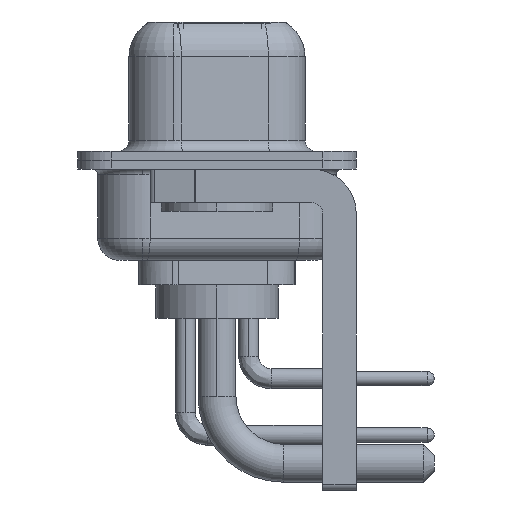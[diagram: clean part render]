
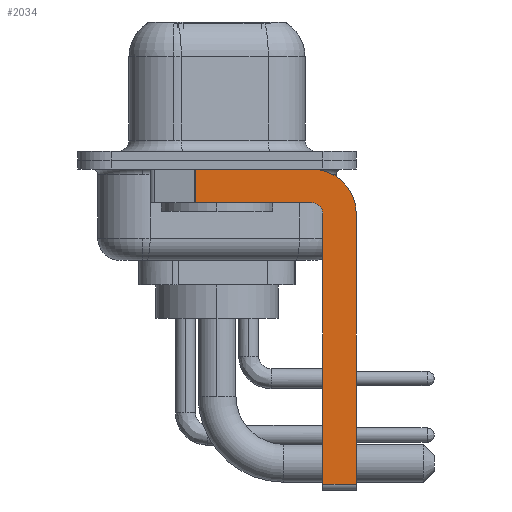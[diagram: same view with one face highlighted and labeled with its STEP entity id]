
A CAD part, left-side view. The second image highlights one B-rep face of the part: STEP entity #2034.
In plain terms, the highlighted planar face has unit normal (-1, 0, 0).
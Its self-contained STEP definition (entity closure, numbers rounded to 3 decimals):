
#954 = CARTESIAN_POINT ( 'NONE',  ( -2.9, -4.25, -2.4 ) ) ;
#1086 = CARTESIAN_POINT ( 'NONE',  ( -2.9, -4.25, -1.9 ) ) ;
#1178 = ORIENTED_EDGE ( 'NONE', *, *, #19862, .F. ) ;
#1414 = CARTESIAN_POINT ( 'NONE',  ( -2.9, -4.25, -2.4 ) ) ;
#1993 = VECTOR ( 'NONE', #14290, 1000. ) ;
#2034 = ADVANCED_FACE ( 'NONE', ( #23791 ), #23675, .F. ) ;
#2101 = CARTESIAN_POINT ( 'NONE',  ( -2.9, 0.978, -1.9 ) ) ;
#2731 = EDGE_CURVE ( 'NONE', #20967, #11376, #6004, .T. ) ;
#3029 = ORIENTED_EDGE ( 'NONE', *, *, #13329, .F. ) ;
#3229 = CARTESIAN_POINT ( 'NONE',  ( -2.9, 0.978, -1.9 ) ) ;
#3939 = VECTOR ( 'NONE', #23721, 1000. ) ;
#5291 = ORIENTED_EDGE ( 'NONE', *, *, #20986, .F. ) ;
#5503 = VERTEX_POINT ( 'NONE', #2101 ) ;
#5798 = CARTESIAN_POINT ( 'NONE',  ( -2.9, 0.978, -0.4 ) ) ;
#6004 = LINE ( 'NONE', #17795, #21801 ) ;
#6081 = CIRCLE ( 'NONE', #11251, 2. ) ;
#6351 = AXIS2_PLACEMENT_3D ( 'NONE', #11247, #16842, #24549 ) ;
#6392 = VERTEX_POINT ( 'NONE', #12825 ) ;
#7117 = VECTOR ( 'NONE', #7435, 1000. ) ;
#7435 = DIRECTION ( 'NONE',  ( 0., 0., -1. ) ) ;
#8086 = CARTESIAN_POINT ( 'NONE',  ( -2.9, -4.75, -14.8 ) ) ;
#8740 = DIRECTION ( 'NONE',  ( 0., 0., -1. ) ) ;
#8925 = LINE ( 'NONE', #16754, #17520 ) ;
#9509 = CARTESIAN_POINT ( 'NONE',  ( -2.9, -6.25, -14.55 ) ) ;
#10780 = VERTEX_POINT ( 'NONE', #21435 ) ;
#10843 = ORIENTED_EDGE ( 'NONE', *, *, #17259, .F. ) ;
#11247 = CARTESIAN_POINT ( 'NONE',  ( -2.9, -4.25, -2.4 ) ) ;
#11251 = AXIS2_PLACEMENT_3D ( 'NONE', #954, #15865, #23703 ) ;
#11376 = VERTEX_POINT ( 'NONE', #11816 ) ;
#11761 = VERTEX_POINT ( 'NONE', #17371 ) ;
#11816 = CARTESIAN_POINT ( 'NONE',  ( -2.9, -4.25, -0.4 ) ) ;
#12672 = LINE ( 'NONE', #3229, #1993 ) ;
#12825 = CARTESIAN_POINT ( 'NONE',  ( -2.9, -4.75, -2.4 ) ) ;
#13329 = EDGE_CURVE ( 'NONE', #11761, #5503, #23602, .T. ) ;
#13817 = CARTESIAN_POINT ( 'NONE',  ( -2.9, -6.25, -2.4 ) ) ;
#13894 = CIRCLE ( 'NONE', #6351, 0.5 ) ;
#14285 = EDGE_LOOP ( 'NONE', ( #14454, #18400, #3029, #19603, #1178, #21521, #5291, #10843 ) ) ;
#14290 = DIRECTION ( 'NONE',  ( 0., 0., -1. ) ) ;
#14454 = ORIENTED_EDGE ( 'NONE', *, *, #2731, .F. ) ;
#14983 = EDGE_CURVE ( 'NONE', #20967, #5503, #12672, .T. ) ;
#15555 = EDGE_CURVE ( 'NONE', #10780, #16162, #8925, .T. ) ;
#15661 = DIRECTION ( 'NONE',  ( 0., 0., 1. ) ) ;
#15865 = DIRECTION ( 'NONE',  ( 1., 0., 0. ) ) ;
#16162 = VERTEX_POINT ( 'NONE', #9509 ) ;
#16754 = CARTESIAN_POINT ( 'NONE',  ( -2.9, -4.25, -14.55 ) ) ;
#16842 = DIRECTION ( 'NONE',  ( -1., 0., 0. ) ) ;
#16985 = LINE ( 'NONE', #24458, #7117 ) ;
#17259 = EDGE_CURVE ( 'NONE', #11376, #19419, #6081, .T. ) ;
#17371 = CARTESIAN_POINT ( 'NONE',  ( -2.9, -4.25, -1.9 ) ) ;
#17518 = LINE ( 'NONE', #8086, #18874 ) ;
#17520 = VECTOR ( 'NONE', #20376, 1000. ) ;
#17795 = CARTESIAN_POINT ( 'NONE',  ( -2.9, 3., -0.4 ) ) ;
#18400 = ORIENTED_EDGE ( 'NONE', *, *, #14983, .T. ) ;
#18874 = VECTOR ( 'NONE', #15661, 1000. ) ;
#19419 = VERTEX_POINT ( 'NONE', #13817 ) ;
#19603 = ORIENTED_EDGE ( 'NONE', *, *, #21392, .F. ) ;
#19800 = DIRECTION ( 'NONE',  ( 0., -1., 0. ) ) ;
#19862 = EDGE_CURVE ( 'NONE', #10780, #6392, #17518, .T. ) ;
#20376 = DIRECTION ( 'NONE',  ( 0., -1., 0. ) ) ;
#20967 = VERTEX_POINT ( 'NONE', #5798 ) ;
#20986 = EDGE_CURVE ( 'NONE', #19419, #16162, #16985, .T. ) ;
#21392 = EDGE_CURVE ( 'NONE', #6392, #11761, #13894, .T. ) ;
#21435 = CARTESIAN_POINT ( 'NONE',  ( -2.9, -4.75, -14.55 ) ) ;
#21521 = ORIENTED_EDGE ( 'NONE', *, *, #15555, .T. ) ;
#21709 = AXIS2_PLACEMENT_3D ( 'NONE', #1414, #22182, #8740 ) ;
#21801 = VECTOR ( 'NONE', #19800, 1000. ) ;
#22182 = DIRECTION ( 'NONE',  ( 1., 0., 0. ) ) ;
#23602 = LINE ( 'NONE', #1086, #3939 ) ;
#23675 = PLANE ( 'NONE',  #21709 ) ;
#23703 = DIRECTION ( 'NONE',  ( 0., 0., -1. ) ) ;
#23721 = DIRECTION ( 'NONE',  ( 0., 1., 0. ) ) ;
#23791 = FACE_OUTER_BOUND ( 'NONE', #14285, .T. ) ;
#24458 = CARTESIAN_POINT ( 'NONE',  ( -2.9, -6.25, -2.4 ) ) ;
#24549 = DIRECTION ( 'NONE',  ( 0., 0., 1. ) ) ;
